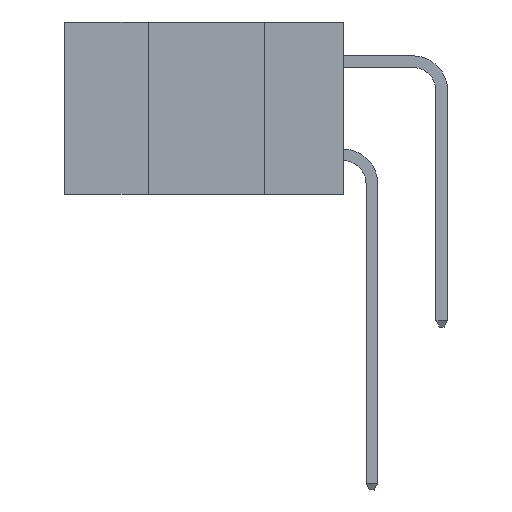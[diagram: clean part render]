
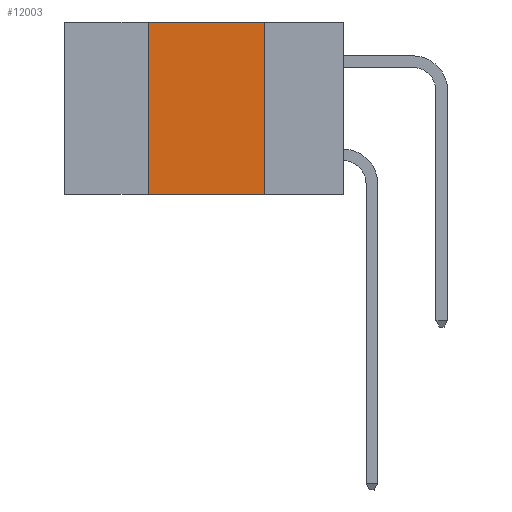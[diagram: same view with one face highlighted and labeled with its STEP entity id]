
A CAD part, left-side view. The second image highlights one B-rep face of the part: STEP entity #12003.
In plain terms, the highlighted planar face has unit normal (-1, 0, 0).
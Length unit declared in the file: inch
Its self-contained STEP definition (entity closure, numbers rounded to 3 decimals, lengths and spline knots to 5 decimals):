
#1974 = ORIENTED_EDGE ( 'NONE', *, *, #9291, .T. ) ;
#2106 = AXIS2_PLACEMENT_3D ( 'NONE', #13053, #15581, #18080 ) ;
#5609 = VECTOR ( 'NONE', #15453, 39.37008 ) ;
#6790 = EDGE_CURVE ( 'NONE', #26431, #14672, #29088, .T. ) ;
#7958 = DIRECTION ( 'NONE',  ( 0., -1., 0. ) ) ;
#8903 = EDGE_CURVE ( 'NONE', #12235, #29955, #25791, .T. ) ;
#9291 = EDGE_CURVE ( 'NONE', #12235, #14672, #24971, .T. ) ;
#10550 = VECTOR ( 'NONE', #23340, 39.37008 ) ;
#10998 = CARTESIAN_POINT ( 'NONE',  ( 0., 0.42, 0. ) ) ;
#11477 = VECTOR ( 'NONE', #24902, 39.37008 ) ;
#12003 = ADVANCED_FACE ( 'NONE', ( #15009 ), #22777, .F. ) ;
#12235 = VERTEX_POINT ( 'NONE', #14619 ) ;
#12553 = CARTESIAN_POINT ( 'NONE',  ( 0., 0.17, 0. ) ) ;
#12813 = CARTESIAN_POINT ( 'NONE',  ( 0., 0.17, -0.37 ) ) ;
#13053 = CARTESIAN_POINT ( 'NONE',  ( 0., 0.6, 0. ) ) ;
#14619 = CARTESIAN_POINT ( 'NONE',  ( 0., 0.42, -0.37 ) ) ;
#14672 = VERTEX_POINT ( 'NONE', #12813 ) ;
#15009 = FACE_OUTER_BOUND ( 'NONE', #17456, .T. ) ;
#15246 = CARTESIAN_POINT ( 'NONE',  ( 0., 0.42, 0. ) ) ;
#15423 = CARTESIAN_POINT ( 'NONE',  ( 0., 0.17, 0. ) ) ;
#15453 = DIRECTION ( 'NONE',  ( 0., -1., 0. ) ) ;
#15581 = DIRECTION ( 'NONE',  ( 1., 0., 0. ) ) ;
#16627 = LINE ( 'NONE', #27898, #5609 ) ;
#17249 = ORIENTED_EDGE ( 'NONE', *, *, #8903, .F. ) ;
#17456 = EDGE_LOOP ( 'NONE', ( #24462, #23588, #17249, #1974 ) ) ;
#18080 = DIRECTION ( 'NONE',  ( 0., 0., -1. ) ) ;
#20390 = EDGE_CURVE ( 'NONE', #29955, #26431, #16627, .T. ) ;
#22777 = PLANE ( 'NONE',  #2106 ) ;
#23340 = DIRECTION ( 'NONE',  ( 0., 0., 1. ) ) ;
#23588 = ORIENTED_EDGE ( 'NONE', *, *, #20390, .F. ) ;
#24462 = ORIENTED_EDGE ( 'NONE', *, *, #6790, .F. ) ;
#24902 = DIRECTION ( 'NONE',  ( 0., 0., -1. ) ) ;
#24971 = LINE ( 'NONE', #29996, #26928 ) ;
#25791 = LINE ( 'NONE', #10998, #10550 ) ;
#26431 = VERTEX_POINT ( 'NONE', #15423 ) ;
#26928 = VECTOR ( 'NONE', #7958, 39.37008 ) ;
#27898 = CARTESIAN_POINT ( 'NONE',  ( 0., 0.6, 0. ) ) ;
#29088 = LINE ( 'NONE', #12553, #11477 ) ;
#29955 = VERTEX_POINT ( 'NONE', #15246 ) ;
#29996 = CARTESIAN_POINT ( 'NONE',  ( 0., 0.6, -0.37 ) ) ;
